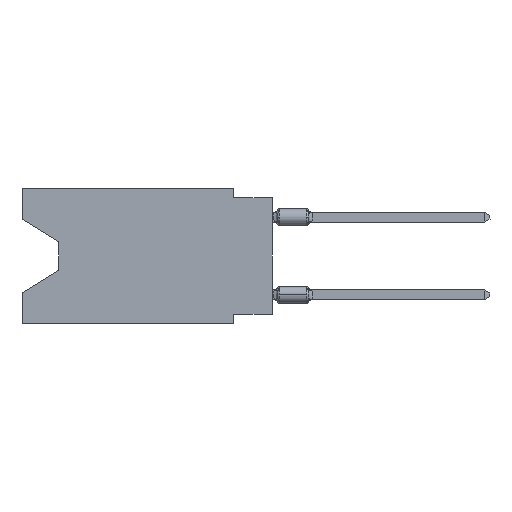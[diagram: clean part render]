
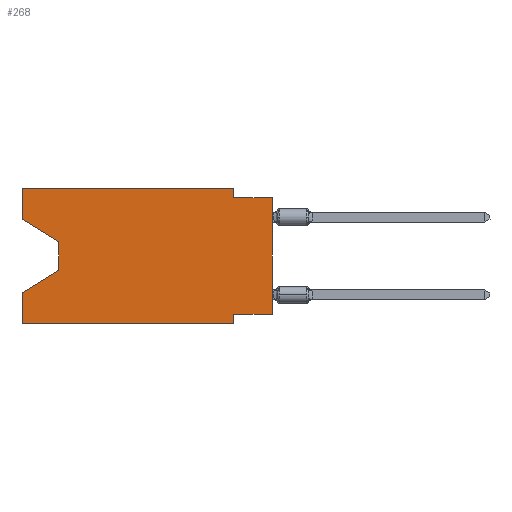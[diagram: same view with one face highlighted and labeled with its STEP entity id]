
A CAD part, left-side view. The second image highlights one B-rep face of the part: STEP entity #268.
In plain terms, the highlighted planar face has unit normal (-1, 0, 0).
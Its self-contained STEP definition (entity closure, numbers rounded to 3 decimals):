
#232 = CARTESIAN_POINT ( 'NONE',  ( 0., 13.97, -5.385 ) ) ;
#268 = ADVANCED_FACE ( 'NONE', ( #9751 ), #606, .F. ) ;
#287 = EDGE_CURVE ( 'NONE', #14342, #16948, #11331, .T. ) ;
#606 = PLANE ( 'NONE',  #14528 ) ;
#690 = CARTESIAN_POINT ( 'NONE',  ( 0., 16.383, 0. ) ) ;
#1017 = DIRECTION ( 'NONE',  ( 0., -1., 0. ) ) ;
#1804 = VECTOR ( 'NONE', #5852, 1000. ) ;
#2253 = CARTESIAN_POINT ( 'NONE',  ( 0., 16.383, 0. ) ) ;
#2440 = CARTESIAN_POINT ( 'NONE',  ( 0., 16.383, 0. ) ) ;
#2574 = CARTESIAN_POINT ( 'NONE',  ( 0., 2.54, -0.635 ) ) ;
#2592 = EDGE_CURVE ( 'NONE', #5792, #3754, #10586, .T. ) ;
#2697 = ORIENTED_EDGE ( 'NONE', *, *, #10806, .F. ) ;
#2741 = CARTESIAN_POINT ( 'NONE',  ( 0., 0., 0. ) ) ;
#3103 = EDGE_CURVE ( 'NONE', #3928, #19509, #13322, .T. ) ;
#3204 = CARTESIAN_POINT ( 'NONE',  ( 0., 16.383, 0. ) ) ;
#3247 = EDGE_CURVE ( 'NONE', #13809, #19509, #9565, .T. ) ;
#3267 = DIRECTION ( 'NONE',  ( 0., -1., 0. ) ) ;
#3284 = VECTOR ( 'NONE', #3267, 1000. ) ;
#3344 = CARTESIAN_POINT ( 'NONE',  ( 0., 16.383, -6.852 ) ) ;
#3492 = DIRECTION ( 'NONE',  ( 0., 0., -1. ) ) ;
#3495 = DIRECTION ( 'NONE',  ( 0., 0., 1. ) ) ;
#3754 = VERTEX_POINT ( 'NONE', #2574 ) ;
#3793 = EDGE_CURVE ( 'NONE', #14468, #7851, #5352, .T. ) ;
#3854 = CARTESIAN_POINT ( 'NONE',  ( 0., 16.383, -2.038 ) ) ;
#3868 = CARTESIAN_POINT ( 'NONE',  ( 0., 13.97, -5.385 ) ) ;
#3902 = CARTESIAN_POINT ( 'NONE',  ( 0., 13.97, -3.505 ) ) ;
#3927 = DIRECTION ( 'NONE',  ( 0., -1., 0. ) ) ;
#3928 = VERTEX_POINT ( 'NONE', #232 ) ;
#4131 = LINE ( 'NONE', #18067, #11670 ) ;
#4326 = VERTEX_POINT ( 'NONE', #19523 ) ;
#4434 = LINE ( 'NONE', #2741, #16802 ) ;
#4608 = VECTOR ( 'NONE', #17498, 1000. ) ;
#5225 = ORIENTED_EDGE ( 'NONE', *, *, #13927, .T. ) ;
#5352 = LINE ( 'NONE', #3854, #6838 ) ;
#5792 = VERTEX_POINT ( 'NONE', #9291 ) ;
#5828 = CARTESIAN_POINT ( 'NONE',  ( 0., 2.54, -8.89 ) ) ;
#5852 = DIRECTION ( 'NONE',  ( 0., 0.855, -0.519 ) ) ;
#6146 = CARTESIAN_POINT ( 'NONE',  ( 0., 0., -8.255 ) ) ;
#6698 = LINE ( 'NONE', #3902, #18678 ) ;
#6740 = EDGE_CURVE ( 'NONE', #16103, #5792, #10005, .T. ) ;
#6838 = VECTOR ( 'NONE', #11309, 1000. ) ;
#6847 = EDGE_CURVE ( 'NONE', #18360, #4326, #4434, .T. ) ;
#7171 = ORIENTED_EDGE ( 'NONE', *, *, #6740, .F. ) ;
#7293 = ORIENTED_EDGE ( 'NONE', *, *, #18383, .F. ) ;
#7698 = ORIENTED_EDGE ( 'NONE', *, *, #3793, .T. ) ;
#7851 = VERTEX_POINT ( 'NONE', #19704 ) ;
#8434 = CARTESIAN_POINT ( 'NONE',  ( 0., 0., -8.255 ) ) ;
#8798 = VECTOR ( 'NONE', #16750, 1000. ) ;
#9212 = EDGE_LOOP ( 'NONE', ( #7698, #5225, #15584, #17115, #17566, #11542, #2697, #15735, #7293, #15175, #7171, #12329 ) ) ;
#9291 = CARTESIAN_POINT ( 'NONE',  ( 0., 2.54, 0. ) ) ;
#9331 = CARTESIAN_POINT ( 'NONE',  ( 0., 0., -0.635 ) ) ;
#9565 = LINE ( 'NONE', #3204, #18660 ) ;
#9751 = FACE_OUTER_BOUND ( 'NONE', #9212, .T. ) ;
#10005 = LINE ( 'NONE', #2253, #11713 ) ;
#10431 = CARTESIAN_POINT ( 'NONE',  ( 0., 16.383, -8.89 ) ) ;
#10586 = LINE ( 'NONE', #15155, #8798 ) ;
#10677 = VECTOR ( 'NONE', #1017, 1000. ) ;
#10806 = EDGE_CURVE ( 'NONE', #18360, #14342, #16387, .T. ) ;
#11075 = CARTESIAN_POINT ( 'NONE',  ( 0., 16.383, -8.89 ) ) ;
#11309 = DIRECTION ( 'NONE',  ( 0., -0.855, -0.519 ) ) ;
#11331 = LINE ( 'NONE', #14314, #18990 ) ;
#11542 = ORIENTED_EDGE ( 'NONE', *, *, #287, .F. ) ;
#11642 = EDGE_CURVE ( 'NONE', #13809, #16948, #18647, .T. ) ;
#11670 = VECTOR ( 'NONE', #16460, 1000. ) ;
#11713 = VECTOR ( 'NONE', #3927, 1000. ) ;
#11989 = DIRECTION ( 'NONE',  ( 0., 0., 1. ) ) ;
#12329 = ORIENTED_EDGE ( 'NONE', *, *, #12537, .F. ) ;
#12537 = EDGE_CURVE ( 'NONE', #14468, #16103, #4131, .T. ) ;
#12912 = DIRECTION ( 'NONE',  ( 1., 0., 0. ) ) ;
#13322 = LINE ( 'NONE', #3868, #1804 ) ;
#13619 = LINE ( 'NONE', #9331, #3284 ) ;
#13809 = VERTEX_POINT ( 'NONE', #10431 ) ;
#13927 = EDGE_CURVE ( 'NONE', #7851, #3928, #6698, .T. ) ;
#14314 = CARTESIAN_POINT ( 'NONE',  ( 0., 2.54, -8.89 ) ) ;
#14342 = VERTEX_POINT ( 'NONE', #15624 ) ;
#14468 = VERTEX_POINT ( 'NONE', #19212 ) ;
#14528 = AXIS2_PLACEMENT_3D ( 'NONE', #690, #12912, #3492 ) ;
#15155 = CARTESIAN_POINT ( 'NONE',  ( 0., 2.54, 0. ) ) ;
#15175 = ORIENTED_EDGE ( 'NONE', *, *, #2592, .F. ) ;
#15584 = ORIENTED_EDGE ( 'NONE', *, *, #3103, .T. ) ;
#15624 = CARTESIAN_POINT ( 'NONE',  ( 0., 2.54, -8.255 ) ) ;
#15735 = ORIENTED_EDGE ( 'NONE', *, *, #6847, .T. ) ;
#16103 = VERTEX_POINT ( 'NONE', #2440 ) ;
#16387 = LINE ( 'NONE', #8434, #4608 ) ;
#16460 = DIRECTION ( 'NONE',  ( 0., 0., 1. ) ) ;
#16750 = DIRECTION ( 'NONE',  ( 0., 0., -1. ) ) ;
#16802 = VECTOR ( 'NONE', #11989, 1000. ) ;
#16948 = VERTEX_POINT ( 'NONE', #5828 ) ;
#17115 = ORIENTED_EDGE ( 'NONE', *, *, #3247, .F. ) ;
#17241 = DIRECTION ( 'NONE',  ( 0., 0., -1. ) ) ;
#17498 = DIRECTION ( 'NONE',  ( 0., 1., 0. ) ) ;
#17566 = ORIENTED_EDGE ( 'NONE', *, *, #11642, .T. ) ;
#18067 = CARTESIAN_POINT ( 'NONE',  ( 0., 16.383, 0. ) ) ;
#18360 = VERTEX_POINT ( 'NONE', #6146 ) ;
#18383 = EDGE_CURVE ( 'NONE', #3754, #4326, #13619, .T. ) ;
#18647 = LINE ( 'NONE', #11075, #10677 ) ;
#18660 = VECTOR ( 'NONE', #3495, 1000. ) ;
#18678 = VECTOR ( 'NONE', #17241, 1000. ) ;
#18897 = DIRECTION ( 'NONE',  ( 0., 0., -1. ) ) ;
#18990 = VECTOR ( 'NONE', #18897, 1000. ) ;
#19212 = CARTESIAN_POINT ( 'NONE',  ( 0., 16.383, -2.038 ) ) ;
#19509 = VERTEX_POINT ( 'NONE', #3344 ) ;
#19523 = CARTESIAN_POINT ( 'NONE',  ( 0., 0., -0.635 ) ) ;
#19704 = CARTESIAN_POINT ( 'NONE',  ( 0., 13.97, -3.505 ) ) ;
